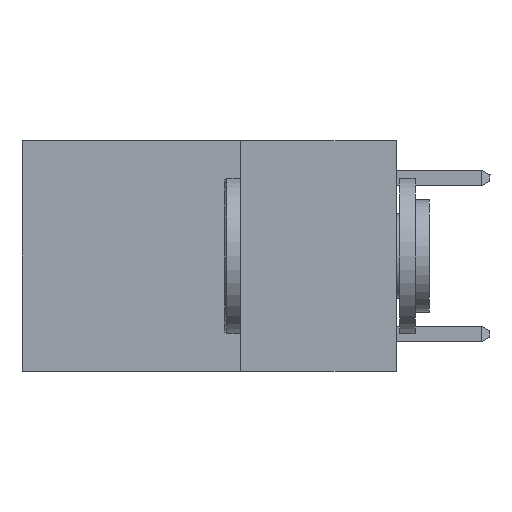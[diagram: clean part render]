
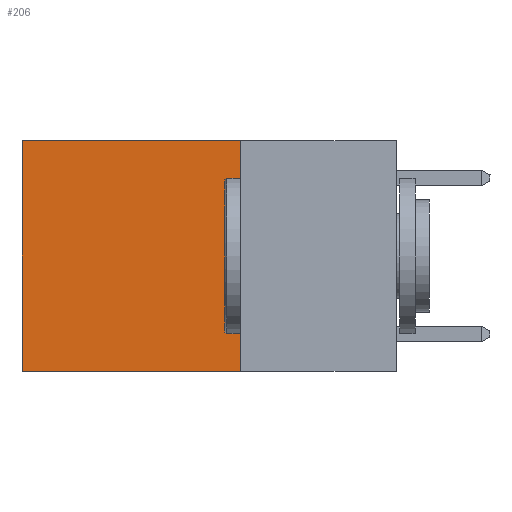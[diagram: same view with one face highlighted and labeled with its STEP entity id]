
A CAD part, left-side view. The second image highlights one B-rep face of the part: STEP entity #206.
In plain terms, the highlighted planar face has unit normal (-1, 0, 0).
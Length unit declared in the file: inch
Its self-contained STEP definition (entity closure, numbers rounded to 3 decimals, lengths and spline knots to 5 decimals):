
#16 = FACE_OUTER_BOUND ( 'NONE', #5658, .T. ) ;
#127 = AXIS2_PLACEMENT_3D ( 'NONE', #10913, #16370, #4115 ) ;
#206 = ADVANCED_FACE ( 'NONE', ( #16 ), #5440, .F. ) ;
#259 = VECTOR ( 'NONE', #7070, 39.37008 ) ;
#953 = CARTESIAN_POINT ( 'NONE',  ( 0.2625, 0.25, 0. ) ) ;
#1632 = CARTESIAN_POINT ( 'NONE',  ( 0.2625, 0.25, 0. ) ) ;
#1633 = CARTESIAN_POINT ( 'NONE',  ( 0.2625, 0.25, -0.37 ) ) ;
#2090 = ORIENTED_EDGE ( 'NONE', *, *, #2313, .T. ) ;
#2313 = EDGE_CURVE ( 'NONE', #3080, #14535, #13194, .T. ) ;
#2796 = LINE ( 'NONE', #1632, #259 ) ;
#3080 = VERTEX_POINT ( 'NONE', #4917 ) ;
#4115 = DIRECTION ( 'NONE',  ( 0., 0., -1. ) ) ;
#4141 = DIRECTION ( 'NONE',  ( 0., 0., -1. ) ) ;
#4262 = DIRECTION ( 'NONE',  ( 0., 1., 0. ) ) ;
#4723 = VERTEX_POINT ( 'NONE', #13605 ) ;
#4917 = CARTESIAN_POINT ( 'NONE',  ( 0.2625, 0.25, 0. ) ) ;
#5113 = EDGE_CURVE ( 'NONE', #6211, #4723, #15998, .T. ) ;
#5440 = PLANE ( 'NONE',  #127 ) ;
#5471 = LINE ( 'NONE', #10942, #6206 ) ;
#5658 = EDGE_LOOP ( 'NONE', ( #13432, #8717, #8232, #2090 ) ) ;
#6206 = VECTOR ( 'NONE', #4141, 39.37008 ) ;
#6211 = VERTEX_POINT ( 'NONE', #1633 ) ;
#6405 = DIRECTION ( 'NONE',  ( 0., 1., 0. ) ) ;
#7070 = DIRECTION ( 'NONE',  ( 0., 0., -1. ) ) ;
#7464 = EDGE_CURVE ( 'NONE', #14535, #4723, #5471, .T. ) ;
#7887 = CARTESIAN_POINT ( 'NONE',  ( 0.2625, 0.6, 0. ) ) ;
#8232 = ORIENTED_EDGE ( 'NONE', *, *, #8553, .F. ) ;
#8553 = EDGE_CURVE ( 'NONE', #3080, #6211, #2796, .T. ) ;
#8717 = ORIENTED_EDGE ( 'NONE', *, *, #5113, .F. ) ;
#8853 = VECTOR ( 'NONE', #6405, 39.37008 ) ;
#10913 = CARTESIAN_POINT ( 'NONE',  ( 0.2625, 0.25, 0. ) ) ;
#10942 = CARTESIAN_POINT ( 'NONE',  ( 0.2625, 0.6, 0. ) ) ;
#11563 = VECTOR ( 'NONE', #4262, 39.37008 ) ;
#13194 = LINE ( 'NONE', #953, #8853 ) ;
#13432 = ORIENTED_EDGE ( 'NONE', *, *, #7464, .T. ) ;
#13605 = CARTESIAN_POINT ( 'NONE',  ( 0.2625, 0.6, -0.37 ) ) ;
#14535 = VERTEX_POINT ( 'NONE', #7887 ) ;
#15998 = LINE ( 'NONE', #17422, #11563 ) ;
#16370 = DIRECTION ( 'NONE',  ( 1., 0., 0. ) ) ;
#17422 = CARTESIAN_POINT ( 'NONE',  ( 0.2625, 0.25, -0.37 ) ) ;
